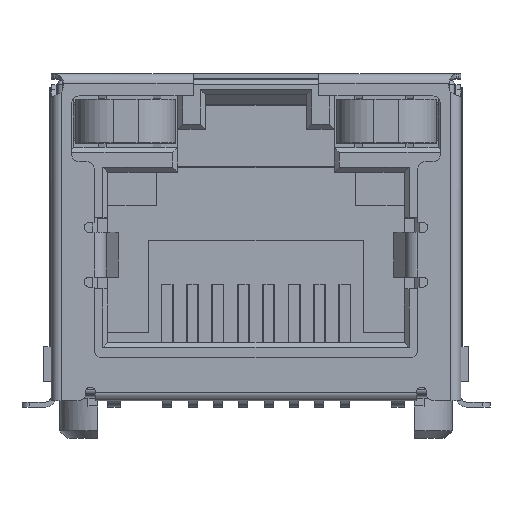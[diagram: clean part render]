
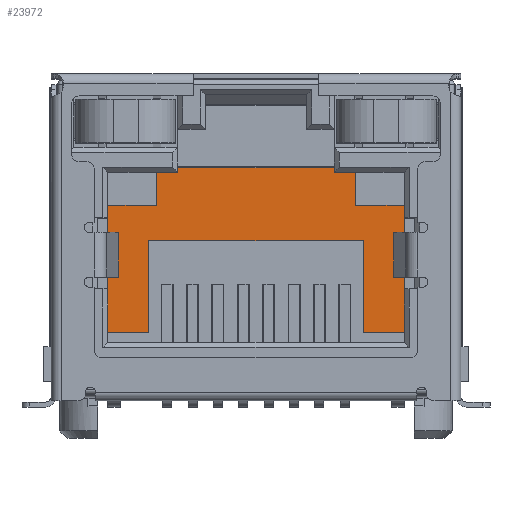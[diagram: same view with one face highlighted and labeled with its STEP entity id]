
A CAD part, top view. The second image highlights one B-rep face of the part: STEP entity #23972.
In plain terms, the highlighted planar face has unit normal (0, 0, 1).
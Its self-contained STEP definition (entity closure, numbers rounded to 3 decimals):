
#29 = EDGE_CURVE ( 'NONE', #26435, #12434, #12468, .T. ) ;
#41 = EDGE_CURVE ( 'NONE', #3665, #7836, #28804, .T. ) ;
#92 = FACE_OUTER_BOUND ( 'NONE', #18284, .T. ) ;
#117 = EDGE_CURVE ( 'NONE', #14528, #7966, #22384, .T. ) ;
#308 = VERTEX_POINT ( 'NONE', #24184 ) ;
#378 = CARTESIAN_POINT ( 'NONE',  ( 2.02, 9.08, -12. ) ) ;
#878 = CARTESIAN_POINT ( 'NONE',  ( 4.825, 9.28, -12. ) ) ;
#1138 = VECTOR ( 'NONE', #14749, 1000. ) ;
#1335 = LINE ( 'NONE', #25475, #5643 ) ;
#1640 = EDGE_CURVE ( 'NONE', #7836, #18270, #27944, .T. ) ;
#1686 = CARTESIAN_POINT ( 'NONE',  ( 12.275, 2.65, -12. ) ) ;
#1770 = VECTOR ( 'NONE', #3225, 1000. ) ;
#1824 = LINE ( 'NONE', #21334, #24629 ) ;
#2810 = LINE ( 'NONE', #23367, #1770 ) ;
#2859 = DIRECTION ( 'NONE',  ( 1., 0., 0. ) ) ;
#2981 = DIRECTION ( 'NONE',  ( 1., 0., 0. ) ) ;
#3025 = CARTESIAN_POINT ( 'NONE',  ( 13.93, 2.65, -12. ) ) ;
#3225 = DIRECTION ( 'NONE',  ( 0., 1., 0. ) ) ;
#3357 = EDGE_CURVE ( 'NONE', #12434, #14528, #17090, .T. ) ;
#3665 = VERTEX_POINT ( 'NONE', #10206 ) ;
#4040 = DIRECTION ( 'NONE',  ( 0., -1., 0. ) ) ;
#4189 = CARTESIAN_POINT ( 'NONE',  ( 13.93, 2.65, -12. ) ) ;
#4218 = VERTEX_POINT ( 'NONE', #12199 ) ;
#4615 = DIRECTION ( 'NONE',  ( -1., 0., 0. ) ) ;
#4776 = VERTEX_POINT ( 'NONE', #3025 ) ;
#4797 = ORIENTED_EDGE ( 'NONE', *, *, #26204, .T. ) ;
#5200 = LINE ( 'NONE', #23345, #12042 ) ;
#5245 = ORIENTED_EDGE ( 'NONE', *, *, #16604, .F. ) ;
#5261 = VERTEX_POINT ( 'NONE', #18860 ) ;
#5266 = DIRECTION ( 'NONE',  ( -1., 0., 0. ) ) ;
#5643 = VECTOR ( 'NONE', #23418, 1000. ) ;
#5943 = VECTOR ( 'NONE', #4040, 1000. ) ;
#6261 = CARTESIAN_POINT ( 'NONE',  ( 2.02, 2.45, -12. ) ) ;
#6468 = PLANE ( 'NONE',  #21699 ) ;
#6743 = EDGE_CURVE ( 'NONE', #4776, #18270, #15852, .T. ) ;
#6960 = CARTESIAN_POINT ( 'NONE',  ( 12.275, 6.35, -12. ) ) ;
#7455 = VECTOR ( 'NONE', #5266, 1000. ) ;
#7773 = EDGE_CURVE ( 'NONE', #16773, #308, #1824, .T. ) ;
#7836 = VERTEX_POINT ( 'NONE', #6960 ) ;
#7966 = VERTEX_POINT ( 'NONE', #10961 ) ;
#8555 = CARTESIAN_POINT ( 'NONE',  ( 2.02, 7.78, -12. ) ) ;
#8682 = VECTOR ( 'NONE', #24900, 1000. ) ;
#8711 = EDGE_CURVE ( 'NONE', #9022, #5261, #23517, .T. ) ;
#9022 = VERTEX_POINT ( 'NONE', #13661 ) ;
#9566 = VECTOR ( 'NONE', #12097, 1000. ) ;
#9686 = VECTOR ( 'NONE', #4615, 1000. ) ;
#10206 = CARTESIAN_POINT ( 'NONE',  ( 3.675, 6.35, -12. ) ) ;
#10720 = ORIENTED_EDGE ( 'NONE', *, *, #3357, .T. ) ;
#10961 = CARTESIAN_POINT ( 'NONE',  ( 2.02, 7.78, -12. ) ) ;
#11052 = ORIENTED_EDGE ( 'NONE', *, *, #14889, .T. ) ;
#11707 = CARTESIAN_POINT ( 'NONE',  ( 2.02, 6.35, -12. ) ) ;
#11748 = VECTOR ( 'NONE', #16176, 1000. ) ;
#11809 = VECTOR ( 'NONE', #20626, 1000. ) ;
#11833 = ORIENTED_EDGE ( 'NONE', *, *, #7773, .T. ) ;
#12042 = VECTOR ( 'NONE', #14121, 1000. ) ;
#12097 = DIRECTION ( 'NONE',  ( -1., 0., 0. ) ) ;
#12138 = ORIENTED_EDGE ( 'NONE', *, *, #14320, .F. ) ;
#12199 = CARTESIAN_POINT ( 'NONE',  ( 11.975, 9.08, -12. ) ) ;
#12434 = VERTEX_POINT ( 'NONE', #20186 ) ;
#12468 = LINE ( 'NONE', #378, #11748 ) ;
#12554 = VERTEX_POINT ( 'NONE', #18682 ) ;
#13325 = ORIENTED_EDGE ( 'NONE', *, *, #41, .T. ) ;
#13361 = EDGE_CURVE ( 'NONE', #21545, #23504, #21091, .T. ) ;
#13601 = ORIENTED_EDGE ( 'NONE', *, *, #20924, .T. ) ;
#13661 = CARTESIAN_POINT ( 'NONE',  ( 11.125, 9.28, -12. ) ) ;
#13713 = CARTESIAN_POINT ( 'NONE',  ( 11.975, 7.78, -12. ) ) ;
#14121 = DIRECTION ( 'NONE',  ( 0., -1., 0. ) ) ;
#14320 = EDGE_CURVE ( 'NONE', #16773, #7966, #24216, .T. ) ;
#14528 = VERTEX_POINT ( 'NONE', #23406 ) ;
#14749 = DIRECTION ( 'NONE',  ( 0., 1., 0. ) ) ;
#14889 = EDGE_CURVE ( 'NONE', #12554, #9022, #2810, .T. ) ;
#15015 = CARTESIAN_POINT ( 'NONE',  ( 2.02, 9.08, -12. ) ) ;
#15018 = ORIENTED_EDGE ( 'NONE', *, *, #117, .T. ) ;
#15485 = DIRECTION ( 'NONE',  ( 0., 0., 1. ) ) ;
#15818 = DIRECTION ( 'NONE',  ( 0., -1., 0. ) ) ;
#15852 = LINE ( 'NONE', #4189, #8682 ) ;
#16169 = LINE ( 'NONE', #26147, #1138 ) ;
#16176 = DIRECTION ( 'NONE',  ( -1., 0., 0. ) ) ;
#16463 = CARTESIAN_POINT ( 'NONE',  ( 2.02, 7.78, -12. ) ) ;
#16604 = EDGE_CURVE ( 'NONE', #21545, #4776, #17720, .T. ) ;
#16773 = VERTEX_POINT ( 'NONE', #20799 ) ;
#17012 = CARTESIAN_POINT ( 'NONE',  ( 13.93, 7.78, -12. ) ) ;
#17069 = VECTOR ( 'NONE', #2859, 1000. ) ;
#17090 = LINE ( 'NONE', #29108, #27368 ) ;
#17626 = CARTESIAN_POINT ( 'NONE',  ( 13.93, 9.08, -12. ) ) ;
#17720 = LINE ( 'NONE', #17626, #5943 ) ;
#18270 = VERTEX_POINT ( 'NONE', #1686 ) ;
#18284 = EDGE_LOOP ( 'NONE', ( #15018, #12138, #11833, #18572, #13325, #26092, #29068, #5245, #18779, #13601, #4797, #11052, #24078, #27940, #19470, #10720 ) ) ;
#18572 = ORIENTED_EDGE ( 'NONE', *, *, #18991, .T. ) ;
#18682 = CARTESIAN_POINT ( 'NONE',  ( 11.125, 9.08, -12. ) ) ;
#18779 = ORIENTED_EDGE ( 'NONE', *, *, #13361, .T. ) ;
#18860 = CARTESIAN_POINT ( 'NONE',  ( 4.825, 9.28, -12. ) ) ;
#18991 = EDGE_CURVE ( 'NONE', #308, #3665, #16169, .T. ) ;
#19470 = ORIENTED_EDGE ( 'NONE', *, *, #29, .T. ) ;
#19573 = DIRECTION ( 'NONE',  ( -1., 0., 0. ) ) ;
#20042 = DIRECTION ( 'NONE',  ( 1., 0., 0. ) ) ;
#20186 = CARTESIAN_POINT ( 'NONE',  ( 3.975, 9.08, -12. ) ) ;
#20626 = DIRECTION ( 'NONE',  ( 0., 1., 0. ) ) ;
#20682 = LINE ( 'NONE', #15015, #25646 ) ;
#20749 = DIRECTION ( 'NONE',  ( 0., -1., 0. ) ) ;
#20799 = CARTESIAN_POINT ( 'NONE',  ( 2.02, 2.65, -12. ) ) ;
#20924 = EDGE_CURVE ( 'NONE', #23504, #4218, #1335, .T. ) ;
#21091 = LINE ( 'NONE', #8555, #9686 ) ;
#21334 = CARTESIAN_POINT ( 'NONE',  ( 2.02, 2.65, -12. ) ) ;
#21545 = VERTEX_POINT ( 'NONE', #17012 ) ;
#21699 = AXIS2_PLACEMENT_3D ( 'NONE', #6261, #15485, #20042 ) ;
#21949 = VECTOR ( 'NONE', #20749, 1000. ) ;
#22055 = EDGE_CURVE ( 'NONE', #5261, #26435, #5200, .T. ) ;
#22384 = LINE ( 'NONE', #16463, #9566 ) ;
#23345 = CARTESIAN_POINT ( 'NONE',  ( 4.825, 2.45, -12. ) ) ;
#23367 = CARTESIAN_POINT ( 'NONE',  ( 11.125, 2.45, -12. ) ) ;
#23406 = CARTESIAN_POINT ( 'NONE',  ( 3.975, 7.78, -12. ) ) ;
#23418 = DIRECTION ( 'NONE',  ( 0., 1., 0. ) ) ;
#23504 = VERTEX_POINT ( 'NONE', #13713 ) ;
#23517 = LINE ( 'NONE', #878, #7455 ) ;
#23972 = ADVANCED_FACE ( 'NONE', ( #92 ), #6468, .T. ) ;
#24078 = ORIENTED_EDGE ( 'NONE', *, *, #8711, .T. ) ;
#24184 = CARTESIAN_POINT ( 'NONE',  ( 3.675, 2.65, -12. ) ) ;
#24216 = LINE ( 'NONE', #25374, #11809 ) ;
#24629 = VECTOR ( 'NONE', #2981, 1000. ) ;
#24900 = DIRECTION ( 'NONE',  ( -1., 0., 0. ) ) ;
#25296 = CARTESIAN_POINT ( 'NONE',  ( 4.825, 9.08, -12. ) ) ;
#25374 = CARTESIAN_POINT ( 'NONE',  ( 2.02, 2.25, -12. ) ) ;
#25475 = CARTESIAN_POINT ( 'NONE',  ( 11.975, 7.78, -12. ) ) ;
#25477 = CARTESIAN_POINT ( 'NONE',  ( 12.275, 2.45, -12. ) ) ;
#25646 = VECTOR ( 'NONE', #19573, 1000. ) ;
#26092 = ORIENTED_EDGE ( 'NONE', *, *, #1640, .T. ) ;
#26147 = CARTESIAN_POINT ( 'NONE',  ( 3.675, 2.45, -12. ) ) ;
#26204 = EDGE_CURVE ( 'NONE', #4218, #12554, #20682, .T. ) ;
#26435 = VERTEX_POINT ( 'NONE', #25296 ) ;
#27368 = VECTOR ( 'NONE', #15818, 1000. ) ;
#27940 = ORIENTED_EDGE ( 'NONE', *, *, #22055, .T. ) ;
#27944 = LINE ( 'NONE', #25477, #21949 ) ;
#28804 = LINE ( 'NONE', #11707, #17069 ) ;
#29068 = ORIENTED_EDGE ( 'NONE', *, *, #6743, .F. ) ;
#29108 = CARTESIAN_POINT ( 'NONE',  ( 3.975, 9.08, -12. ) ) ;
